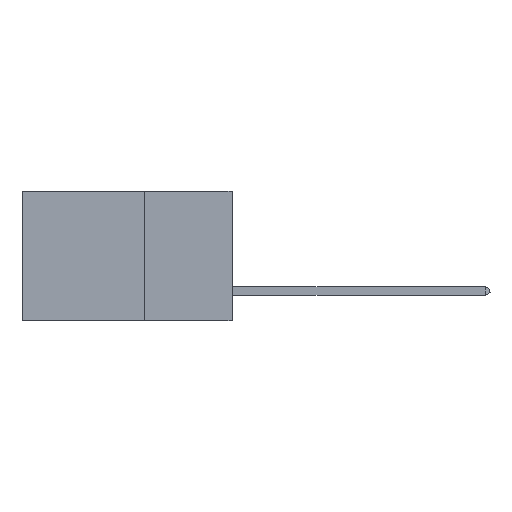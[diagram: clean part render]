
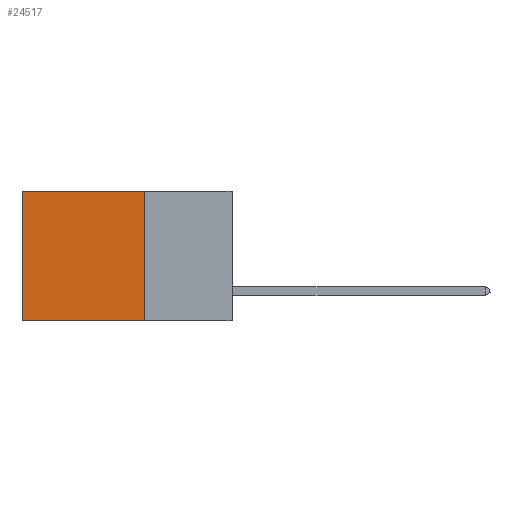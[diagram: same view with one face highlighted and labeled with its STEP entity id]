
A CAD part, left-side view. The second image highlights one B-rep face of the part: STEP entity #24517.
In plain terms, the highlighted planar face has unit normal (-1, 0, 0).
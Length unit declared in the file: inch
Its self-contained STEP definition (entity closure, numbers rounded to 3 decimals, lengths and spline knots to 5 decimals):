
#1330 = ORIENTED_EDGE ( 'NONE', *, *, #20616, .F. ) ;
#3341 = CARTESIAN_POINT ( 'NONE',  ( 0.2875, 0.6, -0.37 ) ) ;
#4001 = ORIENTED_EDGE ( 'NONE', *, *, #31819, .T. ) ;
#5044 = VERTEX_POINT ( 'NONE', #17681 ) ;
#5581 = ORIENTED_EDGE ( 'NONE', *, *, #34123, .T. ) ;
#9554 = VECTOR ( 'NONE', #33647, 39.37008 ) ;
#9811 = EDGE_CURVE ( 'NONE', #42064, #5044, #26701, .T. ) ;
#11069 = CARTESIAN_POINT ( 'NONE',  ( 0.2875, 0.6, 0. ) ) ;
#12858 = CARTESIAN_POINT ( 'NONE',  ( 0.2875, 0.6, 0. ) ) ;
#14921 = LINE ( 'NONE', #12858, #20024 ) ;
#14951 = CARTESIAN_POINT ( 'NONE',  ( 0.2875, 0.25, 0. ) ) ;
#16485 = DIRECTION ( 'NONE',  ( 0., 0., -1. ) ) ;
#17681 = CARTESIAN_POINT ( 'NONE',  ( 0.2875, 0.25, -0.37 ) ) ;
#20024 = VECTOR ( 'NONE', #16485, 39.37008 ) ;
#20253 = CARTESIAN_POINT ( 'NONE',  ( 0.2875, 0.25, 0. ) ) ;
#20616 = EDGE_CURVE ( 'NONE', #5044, #40340, #32828, .T. ) ;
#23880 = FACE_OUTER_BOUND ( 'NONE', #40705, .T. ) ;
#23890 = DIRECTION ( 'NONE',  ( 0., 0., -1. ) ) ;
#24517 = ADVANCED_FACE ( 'NONE', ( #23880 ), #29418, .F. ) ;
#24969 = VECTOR ( 'NONE', #40430, 39.37008 ) ;
#25764 = CARTESIAN_POINT ( 'NONE',  ( 0.2875, 0.25, -0.37 ) ) ;
#26701 = LINE ( 'NONE', #20253, #43895 ) ;
#29418 = PLANE ( 'NONE',  #38736 ) ;
#31511 = ORIENTED_EDGE ( 'NONE', *, *, #9811, .F. ) ;
#31819 = EDGE_CURVE ( 'NONE', #42064, #37165, #38512, .T. ) ;
#32828 = LINE ( 'NONE', #25764, #24969 ) ;
#33052 = CARTESIAN_POINT ( 'NONE',  ( 0.2875, 0.25, 0. ) ) ;
#33647 = DIRECTION ( 'NONE',  ( 0., 1., 0. ) ) ;
#34123 = EDGE_CURVE ( 'NONE', #37165, #40340, #14921, .T. ) ;
#36747 = DIRECTION ( 'NONE',  ( 1., 0., 0. ) ) ;
#37165 = VERTEX_POINT ( 'NONE', #11069 ) ;
#37188 = DIRECTION ( 'NONE',  ( 0., 0., -1. ) ) ;
#37486 = CARTESIAN_POINT ( 'NONE',  ( 0.2875, 0.25, 0. ) ) ;
#38512 = LINE ( 'NONE', #37486, #9554 ) ;
#38736 = AXIS2_PLACEMENT_3D ( 'NONE', #33052, #36747, #37188 ) ;
#40340 = VERTEX_POINT ( 'NONE', #3341 ) ;
#40430 = DIRECTION ( 'NONE',  ( 0., 1., 0. ) ) ;
#40705 = EDGE_LOOP ( 'NONE', ( #5581, #1330, #31511, #4001 ) ) ;
#42064 = VERTEX_POINT ( 'NONE', #14951 ) ;
#43895 = VECTOR ( 'NONE', #23890, 39.37008 ) ;
